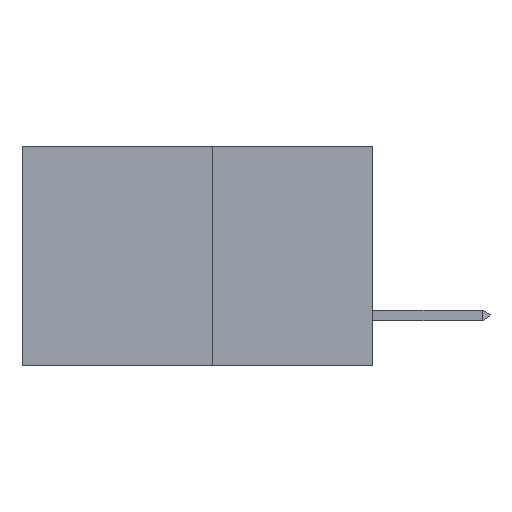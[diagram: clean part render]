
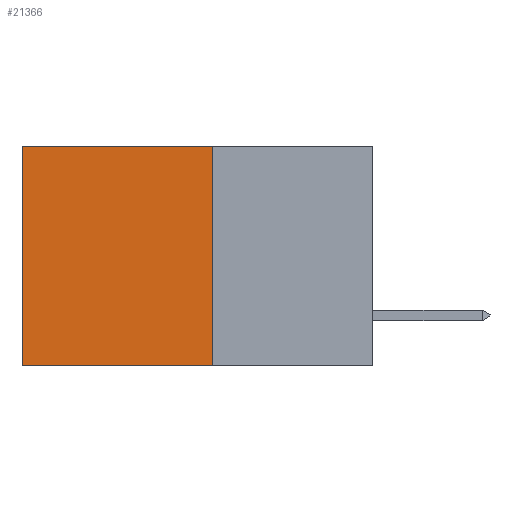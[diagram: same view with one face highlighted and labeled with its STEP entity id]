
A CAD part, left-side view. The second image highlights one B-rep face of the part: STEP entity #21366.
In plain terms, the highlighted planar face has unit normal (-1, 0, 0).
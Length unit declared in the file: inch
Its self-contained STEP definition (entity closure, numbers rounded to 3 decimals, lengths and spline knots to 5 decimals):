
#557 = VERTEX_POINT ( 'NONE', #836 ) ;
#836 = CARTESIAN_POINT ( 'NONE',  ( 0.277, 0.59, 0. ) ) ;
#934 = VERTEX_POINT ( 'NONE', #8274 ) ;
#1059 = ORIENTED_EDGE ( 'NONE', *, *, #27176, .T. ) ;
#2099 = VECTOR ( 'NONE', #18865, 39.37008 ) ;
#2299 = VECTOR ( 'NONE', #11808, 39.37008 ) ;
#3521 = LINE ( 'NONE', #5074, #9140 ) ;
#4752 = FACE_OUTER_BOUND ( 'NONE', #29401, .T. ) ;
#4908 = ORIENTED_EDGE ( 'NONE', *, *, #11115, .F. ) ;
#5074 = CARTESIAN_POINT ( 'NONE',  ( 0.277, 0.27, -0.37 ) ) ;
#8274 = CARTESIAN_POINT ( 'NONE',  ( 0.277, 0.27, 0. ) ) ;
#8524 = LINE ( 'NONE', #16416, #2099 ) ;
#9140 = VECTOR ( 'NONE', #24513, 39.37008 ) ;
#10276 = PLANE ( 'NONE',  #13765 ) ;
#11115 = EDGE_CURVE ( 'NONE', #15813, #21402, #20826, .T. ) ;
#11808 = DIRECTION ( 'NONE',  ( 0., 1., 0. ) ) ;
#12700 = DIRECTION ( 'NONE',  ( 1., 0., 0. ) ) ;
#13765 = AXIS2_PLACEMENT_3D ( 'NONE', #27173, #12700, #29526 ) ;
#15247 = CARTESIAN_POINT ( 'NONE',  ( 0.277, 0.59, -0.37 ) ) ;
#15813 = VERTEX_POINT ( 'NONE', #21840 ) ;
#16416 = CARTESIAN_POINT ( 'NONE',  ( 0.277, 0.27, 0. ) ) ;
#17637 = VECTOR ( 'NONE', #28205, 39.37008 ) ;
#18383 = LINE ( 'NONE', #30562, #17637 ) ;
#18865 = DIRECTION ( 'NONE',  ( 0., 1., 0. ) ) ;
#19093 = CARTESIAN_POINT ( 'NONE',  ( 0.277, 0.27, -0.37 ) ) ;
#20826 = LINE ( 'NONE', #19093, #2299 ) ;
#21366 = ADVANCED_FACE ( 'NONE', ( #4752 ), #10276, .F. ) ;
#21402 = VERTEX_POINT ( 'NONE', #15247 ) ;
#21840 = CARTESIAN_POINT ( 'NONE',  ( 0.277, 0.27, -0.37 ) ) ;
#22715 = ORIENTED_EDGE ( 'NONE', *, *, #29877, .F. ) ;
#24513 = DIRECTION ( 'NONE',  ( 0., 0., -1. ) ) ;
#26147 = ORIENTED_EDGE ( 'NONE', *, *, #26813, .T. ) ;
#26813 = EDGE_CURVE ( 'NONE', #557, #21402, #18383, .T. ) ;
#27173 = CARTESIAN_POINT ( 'NONE',  ( 0.277, 0.27, -0.37 ) ) ;
#27176 = EDGE_CURVE ( 'NONE', #934, #557, #8524, .T. ) ;
#28205 = DIRECTION ( 'NONE',  ( 0., 0., -1. ) ) ;
#29401 = EDGE_LOOP ( 'NONE', ( #26147, #4908, #22715, #1059 ) ) ;
#29526 = DIRECTION ( 'NONE',  ( 0., 0., -1. ) ) ;
#29877 = EDGE_CURVE ( 'NONE', #934, #15813, #3521, .T. ) ;
#30562 = CARTESIAN_POINT ( 'NONE',  ( 0.277, 0.59, -0.37 ) ) ;
